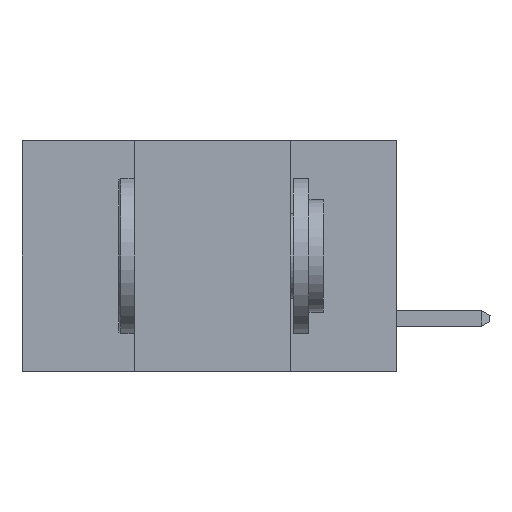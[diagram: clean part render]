
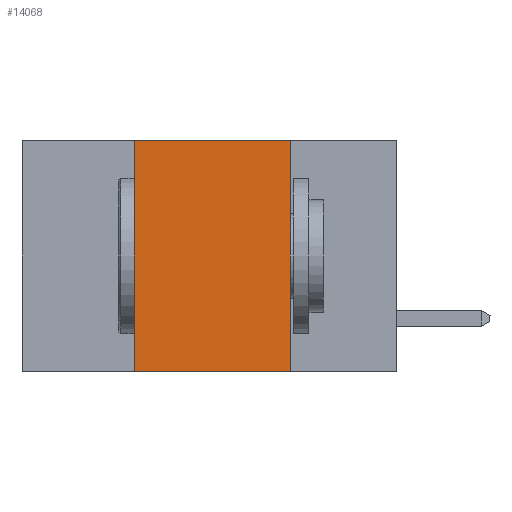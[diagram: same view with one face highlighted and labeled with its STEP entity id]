
A CAD part, left-side view. The second image highlights one B-rep face of the part: STEP entity #14068.
In plain terms, the highlighted planar face has unit normal (-1, 0, 0).
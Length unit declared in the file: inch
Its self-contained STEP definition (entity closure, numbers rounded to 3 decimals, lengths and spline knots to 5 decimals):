
#412 = ORIENTED_EDGE ( 'NONE', *, *, #5815, .F. ) ;
#420 = EDGE_CURVE ( 'NONE', #11252, #10695, #24518, .T. ) ;
#1076 = VECTOR ( 'NONE', #5735, 39.37008 ) ;
#2780 = EDGE_CURVE ( 'NONE', #5851, #10695, #10365, .T. ) ;
#3722 = EDGE_LOOP ( 'NONE', ( #8731, #412, #22200, #13069 ) ) ;
#5735 = DIRECTION ( 'NONE',  ( 0., -1., 0. ) ) ;
#5758 = DIRECTION ( 'NONE',  ( 0., 0., 1. ) ) ;
#5784 = DIRECTION ( 'NONE',  ( 0., 0., -1. ) ) ;
#5815 = EDGE_CURVE ( 'NONE', #16749, #5851, #15079, .T. ) ;
#5838 = CARTESIAN_POINT ( 'NONE',  ( 0., 0.42, 0. ) ) ;
#5851 = VERTEX_POINT ( 'NONE', #5986 ) ;
#5986 = CARTESIAN_POINT ( 'NONE',  ( 0., 0.17, 0. ) ) ;
#7415 = VECTOR ( 'NONE', #18615, 39.37008 ) ;
#7646 = DIRECTION ( 'NONE',  ( 1., 0., 0. ) ) ;
#7713 = CARTESIAN_POINT ( 'NONE',  ( 0., 0.17, -0.37 ) ) ;
#7879 = VECTOR ( 'NONE', #5758, 39.37008 ) ;
#8731 = ORIENTED_EDGE ( 'NONE', *, *, #2780, .F. ) ;
#10365 = LINE ( 'NONE', #11676, #22867 ) ;
#10695 = VERTEX_POINT ( 'NONE', #7713 ) ;
#11252 = VERTEX_POINT ( 'NONE', #14394 ) ;
#11557 = EDGE_CURVE ( 'NONE', #11252, #16749, #14583, .T. ) ;
#11676 = CARTESIAN_POINT ( 'NONE',  ( 0., 0.17, 0. ) ) ;
#13069 = ORIENTED_EDGE ( 'NONE', *, *, #420, .T. ) ;
#14068 = ADVANCED_FACE ( 'NONE', ( #19965 ), #25028, .F. ) ;
#14394 = CARTESIAN_POINT ( 'NONE',  ( 0., 0.42, -0.37 ) ) ;
#14583 = LINE ( 'NONE', #5838, #7879 ) ;
#15079 = LINE ( 'NONE', #25176, #1076 ) ;
#16717 = CARTESIAN_POINT ( 'NONE',  ( 0., 0.6, -0.37 ) ) ;
#16749 = VERTEX_POINT ( 'NONE', #25084 ) ;
#17105 = AXIS2_PLACEMENT_3D ( 'NONE', #25129, #7646, #21039 ) ;
#18615 = DIRECTION ( 'NONE',  ( 0., -1., 0. ) ) ;
#19965 = FACE_OUTER_BOUND ( 'NONE', #3722, .T. ) ;
#21039 = DIRECTION ( 'NONE',  ( 0., 0., -1. ) ) ;
#22200 = ORIENTED_EDGE ( 'NONE', *, *, #11557, .F. ) ;
#22867 = VECTOR ( 'NONE', #5784, 39.37008 ) ;
#24518 = LINE ( 'NONE', #16717, #7415 ) ;
#25028 = PLANE ( 'NONE',  #17105 ) ;
#25084 = CARTESIAN_POINT ( 'NONE',  ( 0., 0.42, 0. ) ) ;
#25129 = CARTESIAN_POINT ( 'NONE',  ( 0., 0.6, 0. ) ) ;
#25176 = CARTESIAN_POINT ( 'NONE',  ( 0., 0.6, 0. ) ) ;
